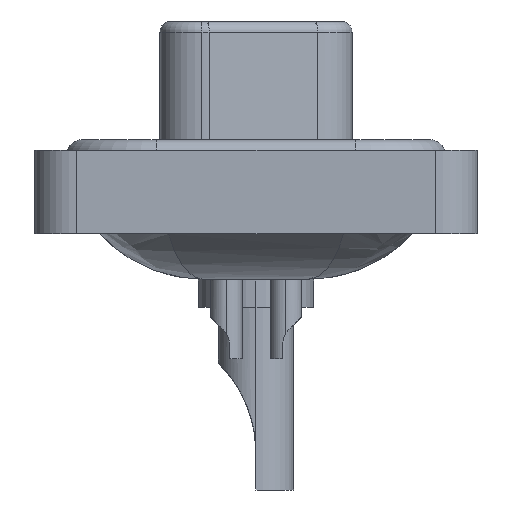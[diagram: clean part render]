
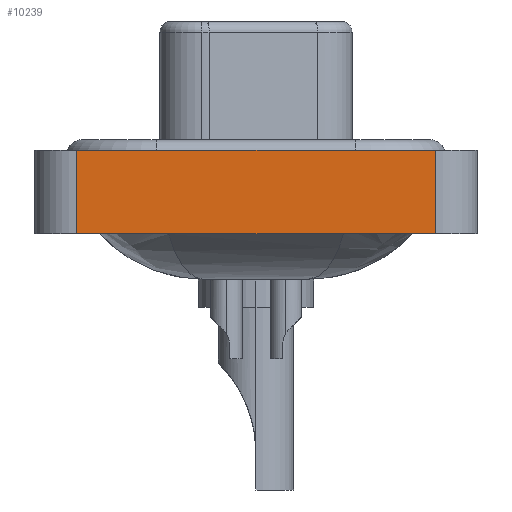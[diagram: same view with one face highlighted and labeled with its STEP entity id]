
A CAD part, left-side view. The second image highlights one B-rep face of the part: STEP entity #10239.
In plain terms, the highlighted planar face has unit normal (-1, 0, 0).
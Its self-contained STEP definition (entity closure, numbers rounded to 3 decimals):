
#875 = CARTESIAN_POINT ( 'NONE',  ( -7.35, 8.55, -3.6 ) ) ;
#1198 = CARTESIAN_POINT ( 'NONE',  ( -7.35, -8.55, 0.4 ) ) ;
#2037 = DIRECTION ( 'NONE',  ( 0., 0., 1. ) ) ;
#3445 = EDGE_CURVE ( 'NONE', #17748, #14014, #18254, .T. ) ;
#4038 = VERTEX_POINT ( 'NONE', #17095 ) ;
#5093 = EDGE_CURVE ( 'NONE', #4038, #11386, #7508, .T. ) ;
#5162 = LINE ( 'NONE', #875, #23818 ) ;
#5795 = LINE ( 'NONE', #22854, #20202 ) ;
#5933 = DIRECTION ( 'NONE',  ( 0., 0., 1. ) ) ;
#5939 = PLANE ( 'NONE',  #20200 ) ;
#7047 = VECTOR ( 'NONE', #10756, 1000. ) ;
#7508 = LINE ( 'NONE', #7885, #8721 ) ;
#7885 = CARTESIAN_POINT ( 'NONE',  ( -7.35, -8.55, -3.6 ) ) ;
#8721 = VECTOR ( 'NONE', #17160, 1000. ) ;
#8877 = EDGE_CURVE ( 'NONE', #11386, #14014, #5795, .T. ) ;
#9062 = ORIENTED_EDGE ( 'NONE', *, *, #5093, .T. ) ;
#9311 = DIRECTION ( 'NONE',  ( -1., 0., 0. ) ) ;
#10239 = ADVANCED_FACE ( 'NONE', ( #23110 ), #5939, .T. ) ;
#10431 = CARTESIAN_POINT ( 'NONE',  ( -7.35, -8.55, 0.4 ) ) ;
#10579 = EDGE_CURVE ( 'NONE', #4038, #17748, #5162, .T. ) ;
#10756 = DIRECTION ( 'NONE',  ( 0., -1., 0. ) ) ;
#11386 = VERTEX_POINT ( 'NONE', #24025 ) ;
#14014 = VERTEX_POINT ( 'NONE', #10431 ) ;
#15129 = CARTESIAN_POINT ( 'NONE',  ( -7.35, 8.55, 0.4 ) ) ;
#15543 = ORIENTED_EDGE ( 'NONE', *, *, #8877, .T. ) ;
#15710 = ORIENTED_EDGE ( 'NONE', *, *, #3445, .F. ) ;
#17095 = CARTESIAN_POINT ( 'NONE',  ( -7.35, 8.55, -3.6 ) ) ;
#17160 = DIRECTION ( 'NONE',  ( 0., -1., 0. ) ) ;
#17748 = VERTEX_POINT ( 'NONE', #15129 ) ;
#18254 = LINE ( 'NONE', #1198, #7047 ) ;
#18945 = CARTESIAN_POINT ( 'NONE',  ( -7.35, -8.55, -3.6 ) ) ;
#19516 = EDGE_LOOP ( 'NONE', ( #15543, #15710, #22232, #9062 ) ) ;
#20200 = AXIS2_PLACEMENT_3D ( 'NONE', #18945, #9311, #2037 ) ;
#20202 = VECTOR ( 'NONE', #5933, 1000. ) ;
#22232 = ORIENTED_EDGE ( 'NONE', *, *, #10579, .F. ) ;
#22854 = CARTESIAN_POINT ( 'NONE',  ( -7.35, -8.55, -3.6 ) ) ;
#23110 = FACE_OUTER_BOUND ( 'NONE', #19516, .T. ) ;
#23818 = VECTOR ( 'NONE', #24190, 1000. ) ;
#24025 = CARTESIAN_POINT ( 'NONE',  ( -7.35, -8.55, -3.6 ) ) ;
#24190 = DIRECTION ( 'NONE',  ( 0., 0., 1. ) ) ;
